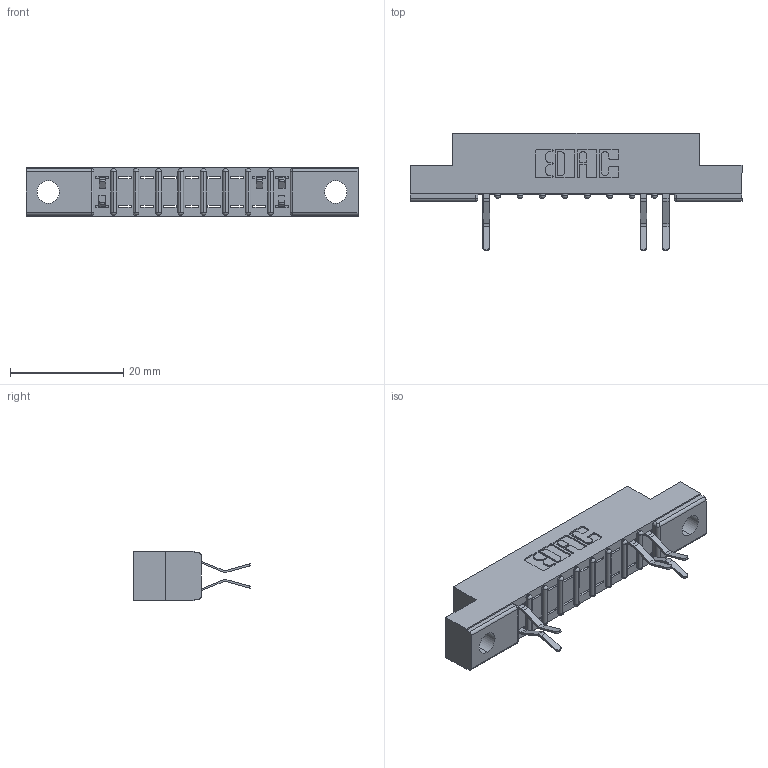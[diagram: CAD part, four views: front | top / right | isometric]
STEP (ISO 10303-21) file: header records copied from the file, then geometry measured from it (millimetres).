
FILE_DESCRIPTION (( 'STEP AP203' ), '1' );
FILE_NAME ('307-018-560-204.STEP', '2018-08-03T23:42:25', ( '' ), ( '' ), 'SwSTEP 2.0', 'SolidWorks 2016', '' );
FILE_SCHEMA (( 'CONFIG_CONTROL_DESIGN' ));
Length unit declared in the file: inch
Products named in the file (3): 307 Part_.156 Dia Mounting Holes; 307-290-001_560; 307-018-560-204
Assembly tree (6 placements, depth 2):
  307-018-560-204
    307 Part_.156 Dia Mounting Holes
    307-290-001_560  x5
Bounding box: 58.67 x 20.73 x 8.71 mm (x, y, z)
Volume: 3571.3 mm3; surface area: 4562.2 mm2
Topology: 6 solids, 6 shells, 522 faces, 1485 edges, 954 vertices
Faces by surface type: plane 327, cylinder 175, sphere 20
Entity records: 12178 total; most frequent: CARTESIAN_POINT 2062, ORIENTED_EDGE 2050, DIRECTION 2013, EDGE_CURVE 1025, LINE 779, VECTOR 779, VERTEX_POINT 666, AXIS2_PLACEMENT_3D 617
